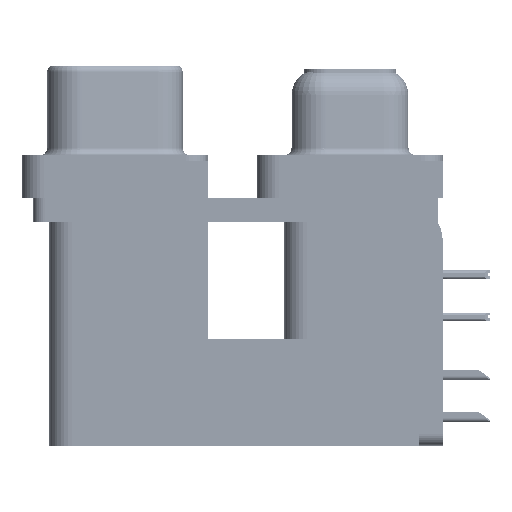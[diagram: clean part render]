
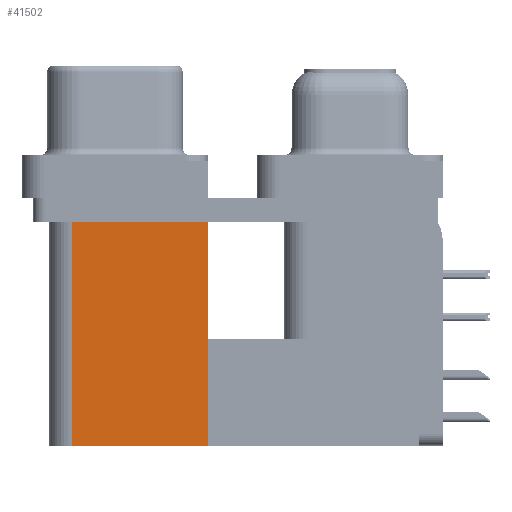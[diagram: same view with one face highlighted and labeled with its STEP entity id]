
A CAD part, left-side view. The second image highlights one B-rep face of the part: STEP entity #41502.
In plain terms, the highlighted planar face has unit normal (-1, 0, 0).
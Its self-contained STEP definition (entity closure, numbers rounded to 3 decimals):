
#580 = VERTEX_POINT ( 'NONE', #29885 ) ;
#1966 = EDGE_CURVE ( 'NONE', #39423, #580, #39206, .T. ) ;
#2920 = EDGE_CURVE ( 'NONE', #39423, #50085, #59977, .T. ) ;
#6024 = CARTESIAN_POINT ( 'NONE',  ( 3.79, 9.6, -19.2 ) ) ;
#7116 = CARTESIAN_POINT ( 'NONE',  ( 3.79, 9.6, -2.5 ) ) ;
#7694 = CARTESIAN_POINT ( 'NONE',  ( 3.79, 18.8, -2.5 ) ) ;
#9506 = ORIENTED_EDGE ( 'NONE', *, *, #23581, .F. ) ;
#13727 = ORIENTED_EDGE ( 'NONE', *, *, #2920, .T. ) ;
#16987 = DIRECTION ( 'NONE',  ( 0., 1., 0. ) ) ;
#19163 = VECTOR ( 'NONE', #36813, 1000. ) ;
#20017 = CARTESIAN_POINT ( 'NONE',  ( 3.79, 9.6, -19.2 ) ) ;
#23581 = EDGE_CURVE ( 'NONE', #580, #26700, #31168, .T. ) ;
#23788 = ORIENTED_EDGE ( 'NONE', *, *, #37392, .T. ) ;
#26700 = VERTEX_POINT ( 'NONE', #7694 ) ;
#29885 = CARTESIAN_POINT ( 'NONE',  ( 3.79, 18.8, -19.2 ) ) ;
#30387 = VECTOR ( 'NONE', #16987, 1000. ) ;
#31168 = LINE ( 'NONE', #52282, #19163 ) ;
#31434 = DIRECTION ( 'NONE',  ( 1., 0., 0. ) ) ;
#32996 = FACE_OUTER_BOUND ( 'NONE', #55395, .T. ) ;
#35360 = VECTOR ( 'NONE', #64577, 1000. ) ;
#36813 = DIRECTION ( 'NONE',  ( 0., 0., 1. ) ) ;
#37392 = EDGE_CURVE ( 'NONE', #50085, #26700, #62221, .T. ) ;
#39206 = LINE ( 'NONE', #20017, #58438 ) ;
#39423 = VERTEX_POINT ( 'NONE', #63940 ) ;
#41502 = ADVANCED_FACE ( 'NONE', ( #32996 ), #53117, .F. ) ;
#43665 = ORIENTED_EDGE ( 'NONE', *, *, #1966, .F. ) ;
#47163 = AXIS2_PLACEMENT_3D ( 'NONE', #6024, #31434, #63327 ) ;
#49729 = DIRECTION ( 'NONE',  ( 0., 1., 0. ) ) ;
#49745 = CARTESIAN_POINT ( 'NONE',  ( 3.79, 9.6, -19.2 ) ) ;
#50085 = VERTEX_POINT ( 'NONE', #57159 ) ;
#52282 = CARTESIAN_POINT ( 'NONE',  ( 3.79, 18.8, -19.2 ) ) ;
#53117 = PLANE ( 'NONE',  #47163 ) ;
#55395 = EDGE_LOOP ( 'NONE', ( #23788, #9506, #43665, #13727 ) ) ;
#57159 = CARTESIAN_POINT ( 'NONE',  ( 3.79, 9.6, -2.5 ) ) ;
#58438 = VECTOR ( 'NONE', #49729, 1000. ) ;
#59977 = LINE ( 'NONE', #49745, #35360 ) ;
#62221 = LINE ( 'NONE', #7116, #30387 ) ;
#63327 = DIRECTION ( 'NONE',  ( 0., 0., -1. ) ) ;
#63940 = CARTESIAN_POINT ( 'NONE',  ( 3.79, 9.6, -19.2 ) ) ;
#64577 = DIRECTION ( 'NONE',  ( 0., 0., 1. ) ) ;
